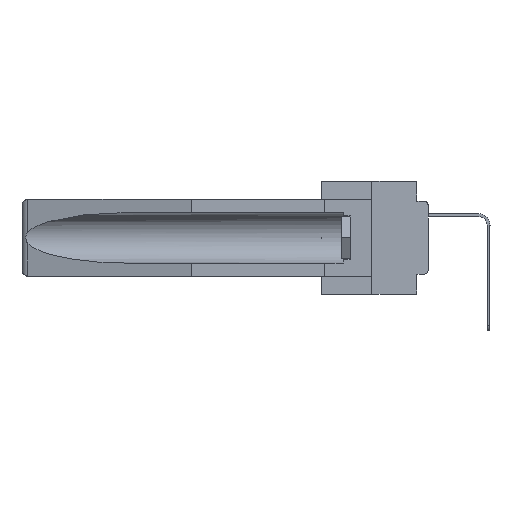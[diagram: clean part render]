
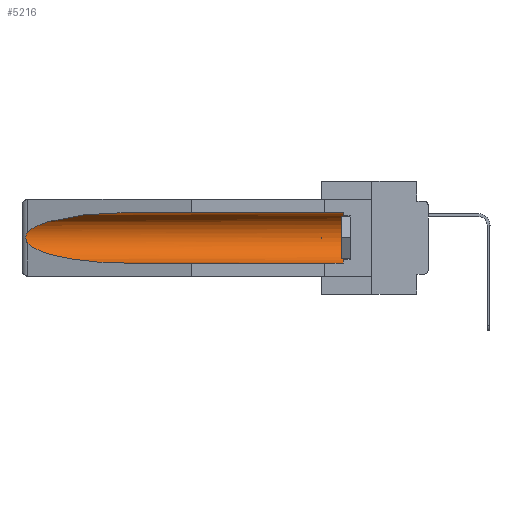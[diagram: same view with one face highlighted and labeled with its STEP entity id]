
A CAD part, left-side view. The second image highlights one B-rep face of the part: STEP entity #5216.
In plain terms, the highlighted cylindrical face has radius 2.857 mm (diameter 5.715 mm), a partial arc.
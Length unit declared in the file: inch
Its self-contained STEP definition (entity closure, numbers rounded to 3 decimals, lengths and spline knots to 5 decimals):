
#14 = DIRECTION ( 'NONE',  ( 0., -1., 0. ) ) ;
#37 = VERTEX_POINT ( 'NONE', #14676 ) ;
#376 = CARTESIAN_POINT ( 'NONE',  ( 0.2673, 1.5327, -0.16383 ) ) ;
#487 = EDGE_LOOP ( 'NONE', ( #28332, #11372, #20216, #21505, #33599, #17983 ) ) ;
#633 = CARTESIAN_POINT ( 'NONE',  ( 0.26537, 1.52718, -0.14972 ) ) ;
#762 = CARTESIAN_POINT ( 'NONE',  ( 0.26597, 1.52961, -0.15275 ) ) ;
#964 = CARTESIAN_POINT ( 'NONE',  ( 0.155, 0.126, -0.059 ) ) ;
#1973 = CARTESIAN_POINT ( 'NONE',  ( 0.155, -0.30754, -0.059 ) ) ;
#2028 = B_SPLINE_CURVE_WITH_KNOTS ( 'NONE', 3,
 ( #633, #762, #36362, #376, #18541, #24130, #15391, #24388, #18415, #24519 ),
 .UNSPECIFIED., .F., .F.,
 ( 4, 2, 2, 2, 4 ),
 ( 0., 0.00029, 0.00058, 0.00087, 0.00117 ),
 .UNSPECIFIED. ) ;
#2100 = CARTESIAN_POINT ( 'NONE',  ( 0.155, 1.07973, -0.059 ) ) ;
#4129 = EDGE_CURVE ( 'NONE', #30803, #37, #2028, .T. ) ;
#5216 = ADVANCED_FACE ( 'NONE', ( #33752 ), #17432, .F. ) ;
#5456 = CARTESIAN_POINT ( 'NONE',  ( 0.155, -0.30754, -0.284 ) ) ;
#6538 = EDGE_CURVE ( 'NONE', #37, #11221, #36576, .T. ) ;
#7374 = CARTESIAN_POINT ( 'NONE',  ( 0.155, 1.07973, -0.284 ) ) ;
#8716 = EDGE_CURVE ( 'NONE', #13308, #11221, #17015, .T. ) ;
#9029 = CARTESIAN_POINT ( 'NONE',  ( 0.26537, 1.52718, -0.14972 ) ) ;
#10552 = DIRECTION ( 'NONE',  ( 0., 1., 0. ) ) ;
#11221 = VERTEX_POINT ( 'NONE', #14571 ) ;
#11372 = ORIENTED_EDGE ( 'NONE', *, *, #4129, .T. ) ;
#11683 = CIRCLE ( 'NONE', #14187, 0.1125 ) ;
#13308 = VERTEX_POINT ( 'NONE', #17825 ) ;
#14187 = AXIS2_PLACEMENT_3D ( 'NONE', #17772, #14, #35116 ) ;
#14374 = EDGE_CURVE ( 'NONE', #37159, #30803, #30857, .T. ) ;
#14571 = CARTESIAN_POINT ( 'NONE',  ( 0.155, 1.07973, -0.284 ) ) ;
#14676 = CARTESIAN_POINT ( 'NONE',  ( 0.26537, 1.52718, -0.19328 ) ) ;
#15391 = CARTESIAN_POINT ( 'NONE',  ( 0.2673, 1.53269, -0.17917 ) ) ;
#15415 = CARTESIAN_POINT ( 'NONE',  ( 0.155, 1.07973, -0.059 ) ) ;
#15535 = CARTESIAN_POINT ( 'NONE',  ( 0.26537, 1.52718, -0.19328 ) ) ;
#16172 = EDGE_CURVE ( 'NONE', #13308, #30868, #11683, .T. ) ;
#17015 = LINE ( 'NONE', #5456, #25887 ) ;
#17149 = CARTESIAN_POINT ( 'NONE',  ( 0.155, -0.30754, -0.1715 ) ) ;
#17432 = CYLINDRICAL_SURFACE ( 'NONE', #28664, 0.1125 ) ;
#17772 = CARTESIAN_POINT ( 'NONE',  ( 0.155, 0.126, -0.1715 ) ) ;
#17825 = CARTESIAN_POINT ( 'NONE',  ( 0.155, 0.126, -0.284 ) ) ;
#17983 = ORIENTED_EDGE ( 'NONE', *, *, #34158, .T. ) ;
#18415 = CARTESIAN_POINT ( 'NONE',  ( 0.26597, 1.5296, -0.19026 ) ) ;
#18541 = CARTESIAN_POINT ( 'NONE',  ( 0.2675, 1.53308, -0.16763 ) ) ;
#20216 = ORIENTED_EDGE ( 'NONE', *, *, #6538, .T. ) ;
#21505 = ORIENTED_EDGE ( 'NONE', *, *, #8716, .F. ) ;
#24130 = CARTESIAN_POINT ( 'NONE',  ( 0.2675, 1.53308, -0.17534 ) ) ;
#24220 = LINE ( 'NONE', #1973, #33545 ) ;
#24388 = CARTESIAN_POINT ( 'NONE',  ( 0.26655, 1.53094, -0.18657 ) ) ;
#24519 = CARTESIAN_POINT ( 'NONE',  ( 0.26537, 1.52718, -0.19328 ) ) ;
#25887 = VECTOR ( 'NONE', #38504, 39.37008 ) ;
#26137 = DIRECTION ( 'NONE',  ( 0., 1., 0. ) ) ;
#26238 = CARTESIAN_POINT ( 'NONE',  ( 0.21114, 1.30732, -0.059 ) ) ;
#26369 = CARTESIAN_POINT ( 'NONE',  ( 0.25451, 1.48313, -0.09465 ) ) ;
#28332 = ORIENTED_EDGE ( 'NONE', *, *, #14374, .T. ) ;
#28664 = AXIS2_PLACEMENT_3D ( 'NONE', #17149, #26137, #36368 ) ;
#29365 = CARTESIAN_POINT ( 'NONE',  ( 0.26537, 1.52718, -0.14972 ) ) ;
#30803 = VERTEX_POINT ( 'NONE', #9029 ) ;
#30857 =( BOUNDED_CURVE ( )  B_SPLINE_CURVE ( 3, ( #2100, #26238, #26369, #29365 ),
 .UNSPECIFIED., .F., .F. ) 
 B_SPLINE_CURVE_WITH_KNOTS ( ( 4, 4 ),
 ( 4.71239, 6.08839 ),
 .UNSPECIFIED. ) 
 CURVE ( )  GEOMETRIC_REPRESENTATION_ITEM ( )  RATIONAL_B_SPLINE_CURVE ( ( 1., 0.848, 0.848, 1. ) ) 
 REPRESENTATION_ITEM ( '' )  );
#30868 = VERTEX_POINT ( 'NONE', #964 ) ;
#33545 = VECTOR ( 'NONE', #10552, 39.37008 ) ;
#33599 = ORIENTED_EDGE ( 'NONE', *, *, #16172, .T. ) ;
#33660 = CARTESIAN_POINT ( 'NONE',  ( 0.25451, 1.48313, -0.24835 ) ) ;
#33752 = FACE_OUTER_BOUND ( 'NONE', #487, .T. ) ;
#34158 = EDGE_CURVE ( 'NONE', #30868, #37159, #24220, .T. ) ;
#35116 = DIRECTION ( 'NONE',  ( 0., 0., 1. ) ) ;
#36362 = CARTESIAN_POINT ( 'NONE',  ( 0.26654, 1.53092, -0.15636 ) ) ;
#36368 = DIRECTION ( 'NONE',  ( 0., 0., 1. ) ) ;
#36375 = CARTESIAN_POINT ( 'NONE',  ( 0.21114, 1.30732, -0.284 ) ) ;
#36576 =( BOUNDED_CURVE ( )  B_SPLINE_CURVE ( 3, ( #15535, #33660, #36375, #7374 ),
 .UNSPECIFIED., .F., .F. ) 
 B_SPLINE_CURVE_WITH_KNOTS ( ( 4, 4 ),
 ( 0.1948, 1.5708 ),
 .UNSPECIFIED. ) 
 CURVE ( )  GEOMETRIC_REPRESENTATION_ITEM ( )  RATIONAL_B_SPLINE_CURVE ( ( 1., 0.848, 0.848, 1. ) ) 
 REPRESENTATION_ITEM ( '' )  );
#37159 = VERTEX_POINT ( 'NONE', #15415 ) ;
#38504 = DIRECTION ( 'NONE',  ( 0., 1., 0. ) ) ;
